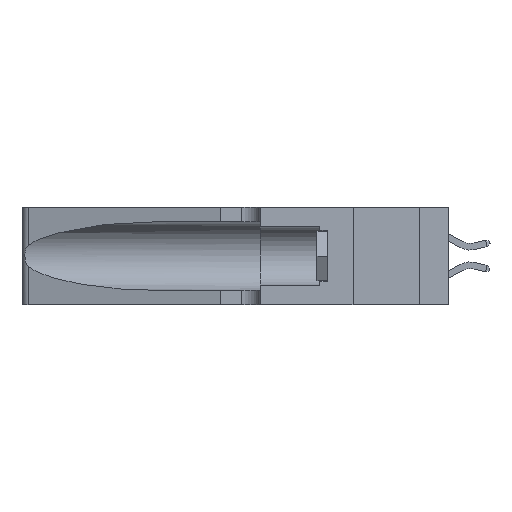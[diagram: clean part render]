
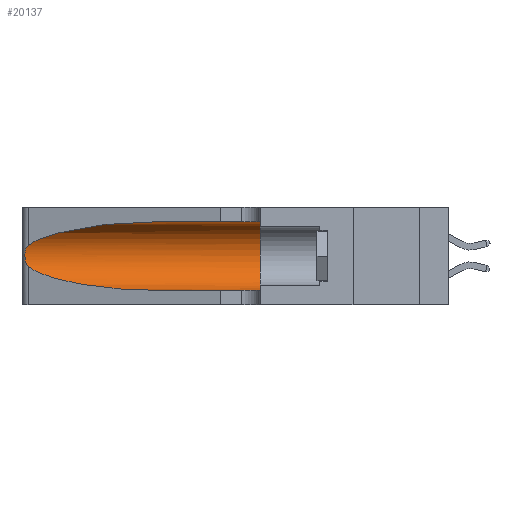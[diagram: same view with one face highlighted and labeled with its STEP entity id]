
A CAD part, left-side view. The second image highlights one B-rep face of the part: STEP entity #20137.
In plain terms, the highlighted cylindrical face has radius 3.308 mm (diameter 6.617 mm), a partial arc.
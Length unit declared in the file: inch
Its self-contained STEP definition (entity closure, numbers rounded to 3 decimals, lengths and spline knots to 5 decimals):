
#9 = CARTESIAN_POINT ( 'NONE',  ( 0.18966, 0.96281, 0.31525 ) ) ;
#725 =( BOUNDED_CURVE ( )  B_SPLINE_CURVE ( 3, ( #25055, #9, #8456, #23047 ),
 .UNSPECIFIED., .F., .F. ) 
 B_SPLINE_CURVE_WITH_KNOTS ( ( 4, 4 ),
 ( 1.5708, 2.84003 ),
 .UNSPECIFIED. ) 
 CURVE ( )  GEOMETRIC_REPRESENTATION_ITEM ( )  RATIONAL_B_SPLINE_CURVE ( ( 1., 0.87, 0.87, 1. ) ) 
 REPRESENTATION_ITEM ( '' )  );
#1520 = CARTESIAN_POINT ( 'NONE',  ( 0.25639, 1.23184, 0.21858 ) ) ;
#1614 = CARTESIAN_POINT ( 'NONE',  ( 0.25555, 1.22993, 0.14849 ) ) ;
#1624 = CARTESIAN_POINT ( 'NONE',  ( 0.2373, 1.15595, 0.08982 ) ) ;
#2277 = EDGE_CURVE ( 'NONE', #2903, #22505, #15301, .T. ) ;
#2460 = CIRCLE ( 'NONE', #6415, 0.13025 ) ;
#2903 = VERTEX_POINT ( 'NONE', #9685 ) ;
#3180 = VERTEX_POINT ( 'NONE', #21011 ) ;
#3395 = CARTESIAN_POINT ( 'NONE',  ( 0.1305, 1.61858, 0.05475 ) ) ;
#3646 = CARTESIAN_POINT ( 'NONE',  ( 0.25555, 1.22994, 0.2215 ) ) ;
#4607 = ORIENTED_EDGE ( 'NONE', *, *, #6980, .T. ) ;
#5259 = ORIENTED_EDGE ( 'NONE', *, *, #14512, .F. ) ;
#5581 = DIRECTION ( 'NONE',  ( 0., -1., 0. ) ) ;
#5747 = CARTESIAN_POINT ( 'NONE',  ( 0.25787, 1.23484, 0.2124 ) ) ;
#6259 = LINE ( 'NONE', #13893, #10446 ) ;
#6319 = DIRECTION ( 'NONE',  ( 0., 1., 0. ) ) ;
#6415 = AXIS2_PLACEMENT_3D ( 'NONE', #18802, #6319, #20884 ) ;
#6980 = EDGE_CURVE ( 'NONE', #3180, #7142, #15710, .T. ) ;
#7142 = VERTEX_POINT ( 'NONE', #16336 ) ;
#7525 = ORIENTED_EDGE ( 'NONE', *, *, #7808, .T. ) ;
#7808 = EDGE_CURVE ( 'NONE', #13049, #2903, #725, .T. ) ;
#7826 = CARTESIAN_POINT ( 'NONE',  ( 0.26018, 1.23835, 0.19895 ) ) ;
#8456 = CARTESIAN_POINT ( 'NONE',  ( 0.2373, 1.15595, 0.28018 ) ) ;
#8551 = AXIS2_PLACEMENT_3D ( 'NONE', #17839, #13666, #19939 ) ;
#9685 = CARTESIAN_POINT ( 'NONE',  ( 0.25487, 1.22718, 0.22369 ) ) ;
#9909 = CARTESIAN_POINT ( 'NONE',  ( 0.26075, 1.23896, 0.178 ) ) ;
#10003 = CARTESIAN_POINT ( 'NONE',  ( 0.1305, 0.72297, 0.05475 ) ) ;
#10446 = VECTOR ( 'NONE', #5581, 39.37008 ) ;
#12002 = CARTESIAN_POINT ( 'NONE',  ( 0.25856, 1.23593, 0.16098 ) ) ;
#12399 = CARTESIAN_POINT ( 'NONE',  ( 0.1305, 0.35, 0.31525 ) ) ;
#13049 = VERTEX_POINT ( 'NONE', #18555 ) ;
#13621 = EDGE_CURVE ( 'NONE', #22505, #3180, #25826, .T. ) ;
#13666 = DIRECTION ( 'NONE',  ( 0., -1., 0. ) ) ;
#13893 = CARTESIAN_POINT ( 'NONE',  ( 0.1305, 1.61858, 0.31525 ) ) ;
#14052 = EDGE_LOOP ( 'NONE', ( #7525, #19267, #19922, #4607, #15680, #5259 ) ) ;
#14146 = CARTESIAN_POINT ( 'NONE',  ( 0.25639, 1.23186, 0.15144 ) ) ;
#14512 = EDGE_CURVE ( 'NONE', #13049, #16567, #6259, .T. ) ;
#15301 = B_SPLINE_CURVE_WITH_KNOTS ( 'NONE', 3,
 ( #18228, #3646, #1520, #5747, #20319, #7826, #22409, #9909, #24525, #12002, #26585, #14146, #1614, #16213 ),
 .UNSPECIFIED., .F., .F.,
 ( 4, 2, 2, 2, 2, 2, 4 ),
 ( 0., 0.00027, 0.00053, 0.00107, 0.0016, 0.00187, 0.00214 ),
 .UNSPECIFIED. ) ;
#15680 = ORIENTED_EDGE ( 'NONE', *, *, #16600, .F. ) ;
#15710 = LINE ( 'NONE', #3395, #26117 ) ;
#16213 = CARTESIAN_POINT ( 'NONE',  ( 0.25487, 1.22718, 0.14631 ) ) ;
#16336 = CARTESIAN_POINT ( 'NONE',  ( 0.1305, 0.35, 0.05475 ) ) ;
#16567 = VERTEX_POINT ( 'NONE', #12399 ) ;
#16600 = EDGE_CURVE ( 'NONE', #16567, #7142, #2460, .T. ) ;
#17839 = CARTESIAN_POINT ( 'NONE',  ( 0.1305, 1.61858, 0.185 ) ) ;
#17984 = DIRECTION ( 'NONE',  ( 0., -1., 0. ) ) ;
#18228 = CARTESIAN_POINT ( 'NONE',  ( 0.25487, 1.22718, 0.22369 ) ) ;
#18328 = CARTESIAN_POINT ( 'NONE',  ( 0.25487, 1.22718, 0.14631 ) ) ;
#18555 = CARTESIAN_POINT ( 'NONE',  ( 0.1305, 0.72297, 0.31525 ) ) ;
#18802 = CARTESIAN_POINT ( 'NONE',  ( 0.1305, 0.35, 0.185 ) ) ;
#19267 = ORIENTED_EDGE ( 'NONE', *, *, #2277, .T. ) ;
#19922 = ORIENTED_EDGE ( 'NONE', *, *, #13621, .T. ) ;
#19939 = DIRECTION ( 'NONE',  ( 0., 0., -1. ) ) ;
#20137 = ADVANCED_FACE ( 'NONE', ( #21864 ), #20555, .F. ) ;
#20319 = CARTESIAN_POINT ( 'NONE',  ( 0.25854, 1.2359, 0.20912 ) ) ;
#20555 = CYLINDRICAL_SURFACE ( 'NONE', #8551, 0.13025 ) ;
#20884 = DIRECTION ( 'NONE',  ( 0., 0., 1. ) ) ;
#21011 = CARTESIAN_POINT ( 'NONE',  ( 0.1305, 0.72297, 0.05475 ) ) ;
#21864 = FACE_OUTER_BOUND ( 'NONE', #14052, .T. ) ;
#22409 = CARTESIAN_POINT ( 'NONE',  ( 0.26075, 1.23896, 0.19203 ) ) ;
#22505 = VERTEX_POINT ( 'NONE', #26252 ) ;
#22514 = CARTESIAN_POINT ( 'NONE',  ( 0.18966, 0.96281, 0.05475 ) ) ;
#23047 = CARTESIAN_POINT ( 'NONE',  ( 0.25487, 1.22718, 0.22369 ) ) ;
#24525 = CARTESIAN_POINT ( 'NONE',  ( 0.26017, 1.23833, 0.17102 ) ) ;
#25055 = CARTESIAN_POINT ( 'NONE',  ( 0.1305, 0.72297, 0.31525 ) ) ;
#25826 =( BOUNDED_CURVE ( )  B_SPLINE_CURVE ( 3, ( #18328, #1624, #22514, #10003 ),
 .UNSPECIFIED., .F., .F. ) 
 B_SPLINE_CURVE_WITH_KNOTS ( ( 4, 4 ),
 ( 3.44316, 4.71239 ),
 .UNSPECIFIED. ) 
 CURVE ( )  GEOMETRIC_REPRESENTATION_ITEM ( )  RATIONAL_B_SPLINE_CURVE ( ( 1., 0.87, 0.87, 1. ) ) 
 REPRESENTATION_ITEM ( '' )  );
#26117 = VECTOR ( 'NONE', #17984, 39.37008 ) ;
#26252 = CARTESIAN_POINT ( 'NONE',  ( 0.25487, 1.22718, 0.14631 ) ) ;
#26585 = CARTESIAN_POINT ( 'NONE',  ( 0.25789, 1.23486, 0.15765 ) ) ;
